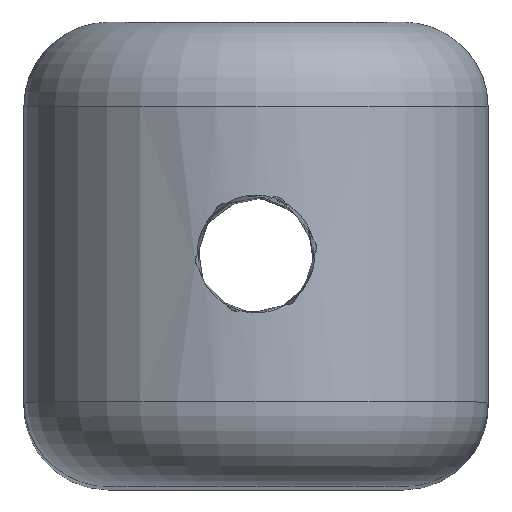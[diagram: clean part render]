
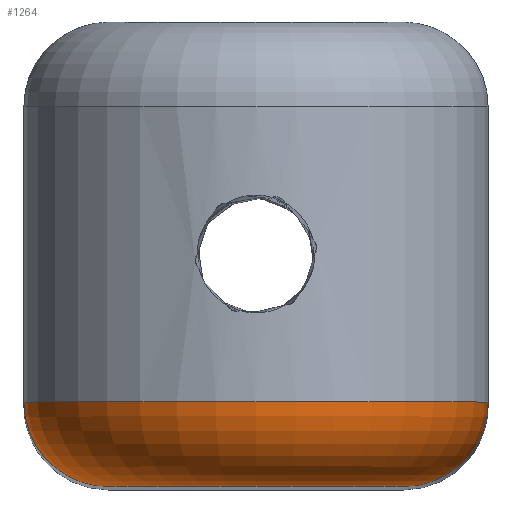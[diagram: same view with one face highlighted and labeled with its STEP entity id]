
A CAD part, top view. The second image highlights one B-rep face of the part: STEP entity #1264.
In plain terms, the highlighted toroidal (fillet/blend) face has major radius 7 mm and minor radius 4 mm.
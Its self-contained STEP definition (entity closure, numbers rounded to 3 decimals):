
#1194=CARTESIAN_POINT('',(-7.,-11.0,99.0));
#1195=VERTEX_POINT('',#1194);
#1196=CARTESIAN_POINT('',(-11.,-7.,99.0));
#1197=VERTEX_POINT('',#1196);
#1198=CARTESIAN_POINT('',(-7.,-7.,99.0));
#1199=DIRECTION('',(0.0,0.0,-1.0));
#1200=DIRECTION('',(0.0,-1.0,0.0));
#1201=AXIS2_PLACEMENT_3D('',#1198,#1199,#1200);
#1202=CIRCLE('',#1201,4.0);
#1203=EDGE_CURVE('',#1195,#1197,#1202,.T.);
#1231=CARTESIAN_POINT('',(0.,-7.,99.0));
#1232=DIRECTION('',(0.0,1.0,0.0));
#1233=DIRECTION('',(0.0,0.0,1.0));
#1234=AXIS2_PLACEMENT_3D('',#1231,#1232,#1233);
#1235=TOROIDAL_SURFACE('',#1234,7.,4.0);
#1236=CARTESIAN_POINT('',(7.,-11.0,99.0));
#1237=VERTEX_POINT('',#1236);
#1238=CARTESIAN_POINT('',(11.,-7.,99.0));
#1239=VERTEX_POINT('',#1238);
#1240=CARTESIAN_POINT('',(7.,-7.,99.0));
#1241=DIRECTION('',(0.0,0.0,1.0));
#1242=DIRECTION('',(0.0,-1.0,0.0));
#1243=AXIS2_PLACEMENT_3D('',#1240,#1241,#1242);
#1244=CIRCLE('',#1243,4.0);
#1245=EDGE_CURVE('',#1237,#1239,#1244,.T.);
#1246=ORIENTED_EDGE('',*,*,#1245,.T.);
#1247=CARTESIAN_POINT('',(0.,-7.,99.0));
#1248=DIRECTION('',(0.0,-1.0,0.0));
#1249=DIRECTION('',(0.0,0.0,1.0));
#1250=AXIS2_PLACEMENT_3D('',#1247,#1248,#1249);
#1251=CIRCLE('',#1250,11.0);
#1252=EDGE_CURVE('',#1239,#1197,#1251,.T.);
#1253=ORIENTED_EDGE('',*,*,#1252,.T.);
#1254=ORIENTED_EDGE('',*,*,#1203,.F.);
#1255=CARTESIAN_POINT('',(0.,-11.0,99.0));
#1256=DIRECTION('',(0.0,1.0,0.0));
#1257=DIRECTION('',(0.0,0.0,1.0));
#1258=AXIS2_PLACEMENT_3D('',#1255,#1256,#1257);
#1259=CIRCLE('',#1258,7.);
#1260=EDGE_CURVE('',#1195,#1237,#1259,.T.);
#1261=ORIENTED_EDGE('',*,*,#1260,.T.);
#1262=EDGE_LOOP('',(#1246,#1253,#1254,#1261));
#1263=FACE_OUTER_BOUND('',#1262,.T.);
#1264=ADVANCED_FACE('',(#1263),#1235,.T.);
